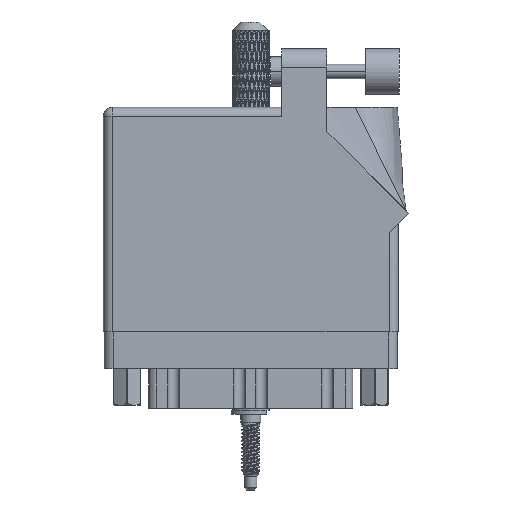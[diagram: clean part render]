
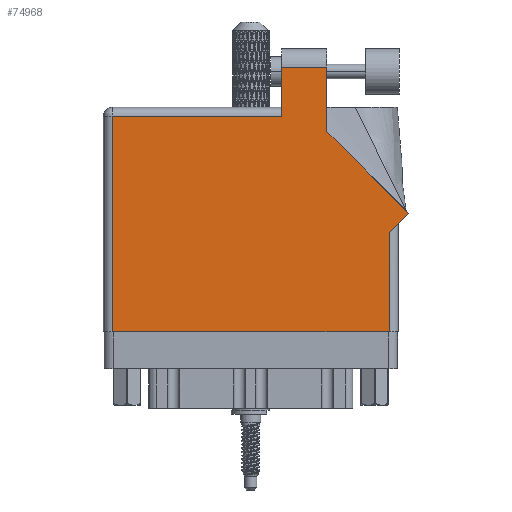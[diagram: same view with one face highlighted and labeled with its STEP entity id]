
A CAD part, front view. The second image highlights one B-rep face of the part: STEP entity #74968.
In plain terms, the highlighted face is planar.
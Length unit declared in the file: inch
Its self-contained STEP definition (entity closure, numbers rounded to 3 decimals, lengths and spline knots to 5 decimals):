
#879 = ORIENTED_EDGE ( 'NONE', *, *, #52124, .T. ) ;
#1694 = VERTEX_POINT ( 'NONE', #41091 ) ;
#2427 = VECTOR ( 'NONE', #89067, 39.37008 ) ;
#4826 = DIRECTION ( 'NONE',  ( -1., 0., 0. ) ) ;
#6605 = EDGE_CURVE ( 'NONE', #33728, #24191, #42669, .T. ) ;
#6637 = DIRECTION ( 'NONE',  ( -1., 0., 0. ) ) ;
#6863 = LINE ( 'NONE', #34350, #51143 ) ;
#9205 = ORIENTED_EDGE ( 'NONE', *, *, #109798, .T. ) ;
#12443 = EDGE_CURVE ( 'NONE', #1694, #32131, #67264, .T. ) ;
#14653 = CARTESIAN_POINT ( 'NONE',  ( 1.217, 1.805, 0. ) ) ;
#14770 = DIRECTION ( 'NONE',  ( -0.707, 0.707, 0. ) ) ;
#16038 = PLANE ( 'NONE',  #85427 ) ;
#17353 = ORIENTED_EDGE ( 'NONE', *, *, #101376, .T. ) ;
#20009 = ORIENTED_EDGE ( 'NONE', *, *, #12443, .T. ) ;
#20689 = EDGE_CURVE ( 'NONE', #111001, #1694, #28404, .T. ) ;
#21094 = CARTESIAN_POINT ( 'NONE',  ( 2.08071, 0.80771, 0. ) ) ;
#23176 = DIRECTION ( 'NONE',  ( 0.707, 0.707, 0. ) ) ;
#24191 = VERTEX_POINT ( 'NONE', #56451 ) ;
#27047 = VERTEX_POINT ( 'NONE', #31465 ) ;
#28404 = LINE ( 'NONE', #106249, #2427 ) ;
#30368 = LINE ( 'NONE', #91040, #65517 ) ;
#30655 = CARTESIAN_POINT ( 'NONE',  ( 2.01, 0.737, 0. ) ) ;
#31465 = CARTESIAN_POINT ( 'NONE',  ( 1.524, 1.36442, 0. ) ) ;
#31995 = EDGE_CURVE ( 'NONE', #27047, #43659, #30368, .T. ) ;
#32131 = VERTEX_POINT ( 'NONE', #35722 ) ;
#33728 = VERTEX_POINT ( 'NONE', #100515 ) ;
#34350 = CARTESIAN_POINT ( 'NONE',  ( 1.217, 1.53, 0. ) ) ;
#34384 = DIRECTION ( 'NONE',  ( -1., 0., 0. ) ) ;
#35722 = CARTESIAN_POINT ( 'NONE',  ( 2.08071, 0.80771, 0. ) ) ;
#41091 = CARTESIAN_POINT ( 'NONE',  ( 1.948, 0.675, 0. ) ) ;
#42669 = LINE ( 'NONE', #76452, #87344 ) ;
#42925 = CARTESIAN_POINT ( 'NONE',  ( 0., 1.53, 0. ) ) ;
#43659 = VERTEX_POINT ( 'NONE', #76851 ) ;
#48731 = EDGE_CURVE ( 'NONE', #24191, #82272, #94087, .T. ) ;
#50752 = CARTESIAN_POINT ( 'NONE',  ( 0., 0., 0. ) ) ;
#51143 = VECTOR ( 'NONE', #59521, 39.37008 ) ;
#52124 = EDGE_CURVE ( 'NONE', #111268, #33728, #6863, .T. ) ;
#56373 = LINE ( 'NONE', #83264, #59800 ) ;
#56451 = CARTESIAN_POINT ( 'NONE',  ( 0.062, 1.468, 0. ) ) ;
#58888 = ORIENTED_EDGE ( 'NONE', *, *, #6605, .T. ) ;
#59521 = DIRECTION ( 'NONE',  ( 0., -1., 0. ) ) ;
#59800 = VECTOR ( 'NONE', #4826, 39.37008 ) ;
#59991 = ORIENTED_EDGE ( 'NONE', *, *, #48731, .T. ) ;
#65517 = VECTOR ( 'NONE', #92159, 39.37008 ) ;
#65876 = EDGE_LOOP ( 'NONE', ( #69296, #17353, #879, #58888, #59991, #76031, #94139, #20009, #9205 ) ) ;
#67264 = LINE ( 'NONE', #30655, #108466 ) ;
#67278 = CARTESIAN_POINT ( 'NONE',  ( 0.062, 0., 0. ) ) ;
#68336 = CARTESIAN_POINT ( 'NONE',  ( 0.062, 0., 0. ) ) ;
#69296 = ORIENTED_EDGE ( 'NONE', *, *, #31995, .T. ) ;
#74968 = ADVANCED_FACE ( 'NONE', ( #94467 ), #16038, .F. ) ;
#75434 = LINE ( 'NONE', #21094, #93134 ) ;
#75923 = DIRECTION ( 'NONE',  ( 1., 0., 0. ) ) ;
#76031 = ORIENTED_EDGE ( 'NONE', *, *, #98233, .T. ) ;
#76452 = CARTESIAN_POINT ( 'NONE',  ( 0., 1.468, 0. ) ) ;
#76851 = CARTESIAN_POINT ( 'NONE',  ( 1.524, 1.805, 0. ) ) ;
#79721 = VECTOR ( 'NONE', #75923, 39.37008 ) ;
#82272 = VERTEX_POINT ( 'NONE', #67278 ) ;
#83264 = CARTESIAN_POINT ( 'NONE',  ( 1.217, 1.805, 0. ) ) ;
#85427 = AXIS2_PLACEMENT_3D ( 'NONE', #42925, #112792, #34384 ) ;
#87344 = VECTOR ( 'NONE', #6637, 39.37008 ) ;
#89067 = DIRECTION ( 'NONE',  ( 0., 1., 0. ) ) ;
#91040 = CARTESIAN_POINT ( 'NONE',  ( 1.524, 1.36442, 0. ) ) ;
#92159 = DIRECTION ( 'NONE',  ( 0., 1., 0. ) ) ;
#93134 = VECTOR ( 'NONE', #14770, 39.37008 ) ;
#94087 = LINE ( 'NONE', #68336, #112953 ) ;
#94139 = ORIENTED_EDGE ( 'NONE', *, *, #20689, .T. ) ;
#94245 = LINE ( 'NONE', #50752, #79721 ) ;
#94467 = FACE_OUTER_BOUND ( 'NONE', #65876, .T. ) ;
#98233 = EDGE_CURVE ( 'NONE', #82272, #111001, #94245, .T. ) ;
#100515 = CARTESIAN_POINT ( 'NONE',  ( 1.217, 1.468, 0. ) ) ;
#101376 = EDGE_CURVE ( 'NONE', #43659, #111268, #56373, .T. ) ;
#101540 = DIRECTION ( 'NONE',  ( 0., -1., 0. ) ) ;
#106249 = CARTESIAN_POINT ( 'NONE',  ( 1.948, 0.737, 0. ) ) ;
#108466 = VECTOR ( 'NONE', #23176, 39.37008 ) ;
#109798 = EDGE_CURVE ( 'NONE', #32131, #27047, #75434, .T. ) ;
#110553 = CARTESIAN_POINT ( 'NONE',  ( 1.948, 0., 0. ) ) ;
#111001 = VERTEX_POINT ( 'NONE', #110553 ) ;
#111268 = VERTEX_POINT ( 'NONE', #14653 ) ;
#112792 = DIRECTION ( 'NONE',  ( 0., 0., -1. ) ) ;
#112953 = VECTOR ( 'NONE', #101540, 39.37008 ) ;
